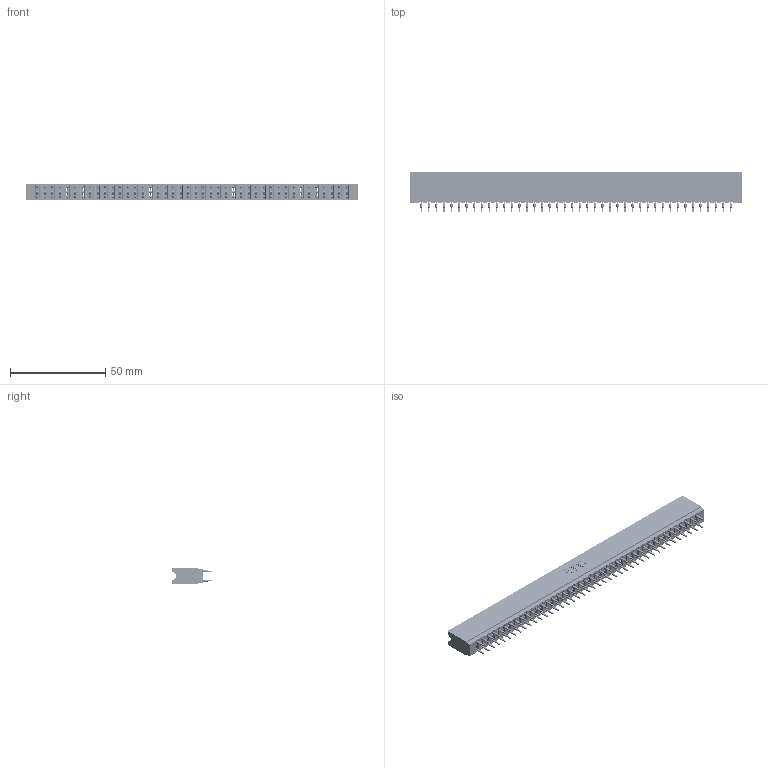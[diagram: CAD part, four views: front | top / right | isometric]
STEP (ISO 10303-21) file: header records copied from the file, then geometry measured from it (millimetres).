
FILE_DESCRIPTION (( 'STEP AP203' ), '1' );
FILE_NAME ('737-084-560-206.STEP', '2026-03-06T02:26:32', ( '' ), ( '' ), 'SwSTEP 2.0', 'SolidWorks 2023', '' );
FILE_SCHEMA (( 'CONFIG_CONTROL_DESIGN' ));
Length unit declared in the file: millimetre
Products named in the file (3): 737 Part_Insulator Option - 06; 737-084-560-206; 745-292-001_560
Assembly tree (85 placements, depth 2):
  737-084-560-206
    737 Part_Insulator Option - 06
    745-292-001_560  x84
Bounding box: 174.29 x 21.22 x 8.89 mm (x, y, z)
Volume: 17456.2 mm3; surface area: 27236.9 mm2
Topology: 85 solids, 85 shells, 8411 faces, 23021 edges, 14618 vertices
Faces by surface type: plane 4381, cylinder 1846, bspline 1680, torus 504
Entity records: 72404 total; most frequent: CARTESIAN_POINT 13074, ORIENTED_EDGE 12510, DIRECTION 10923, EDGE_CURVE 6255, LINE 5813, VECTOR 5813, VERTEX_POINT 3994, AXIS2_PLACEMENT_3D 2555
